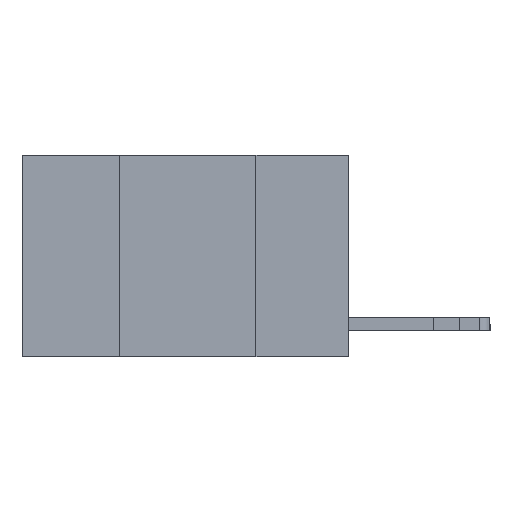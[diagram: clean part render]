
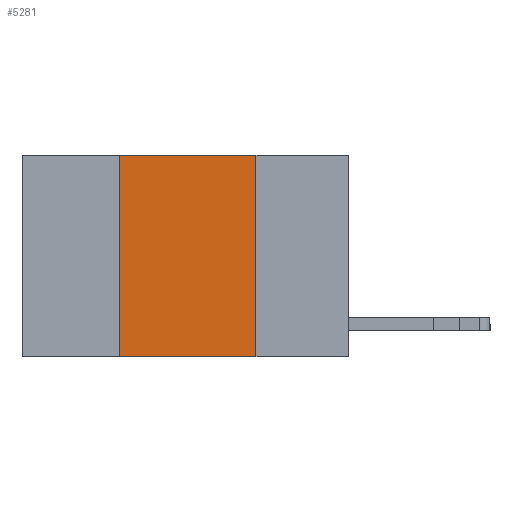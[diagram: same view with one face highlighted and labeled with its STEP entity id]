
A CAD part, left-side view. The second image highlights one B-rep face of the part: STEP entity #5281.
In plain terms, the highlighted planar face has unit normal (-1, 0, 0).
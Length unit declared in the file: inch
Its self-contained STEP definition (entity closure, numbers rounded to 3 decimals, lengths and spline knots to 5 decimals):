
#554 = CARTESIAN_POINT ( 'NONE',  ( 0., 0.42, 0. ) ) ;
#626 = CARTESIAN_POINT ( 'NONE',  ( 0., 0.42, 0. ) ) ;
#970 = ORIENTED_EDGE ( 'NONE', *, *, #9304, .F. ) ;
#1536 = DIRECTION ( 'NONE',  ( 0., -1., 0. ) ) ;
#3220 = EDGE_CURVE ( 'NONE', #19806, #18971, #14054, .T. ) ;
#4281 = LINE ( 'NONE', #626, #7802 ) ;
#4770 = ORIENTED_EDGE ( 'NONE', *, *, #15512, .T. ) ;
#5281 = ADVANCED_FACE ( 'NONE', ( #21952 ), #5828, .F. ) ;
#5628 = CARTESIAN_POINT ( 'NONE',  ( 0., 0.6, 0. ) ) ;
#5828 = PLANE ( 'NONE',  #13904 ) ;
#6828 = CARTESIAN_POINT ( 'NONE',  ( 0., 0.17, -0.37 ) ) ;
#6884 = VERTEX_POINT ( 'NONE', #6828 ) ;
#6937 = VECTOR ( 'NONE', #21202, 39.37008 ) ;
#7802 = VECTOR ( 'NONE', #11305, 39.37008 ) ;
#9304 = EDGE_CURVE ( 'NONE', #18971, #6884, #22130, .T. ) ;
#10269 = LINE ( 'NONE', #20995, #11437 ) ;
#10493 = EDGE_CURVE ( 'NONE', #11701, #19806, #4281, .T. ) ;
#10815 = ORIENTED_EDGE ( 'NONE', *, *, #3220, .F. ) ;
#11289 = CARTESIAN_POINT ( 'NONE',  ( 0., 0.17, 0. ) ) ;
#11305 = DIRECTION ( 'NONE',  ( 0., 0., 1. ) ) ;
#11437 = VECTOR ( 'NONE', #1536, 39.37008 ) ;
#11701 = VERTEX_POINT ( 'NONE', #17473 ) ;
#13904 = AXIS2_PLACEMENT_3D ( 'NONE', #20468, #15609, #16902 ) ;
#14054 = LINE ( 'NONE', #5628, #6937 ) ;
#15512 = EDGE_CURVE ( 'NONE', #11701, #6884, #10269, .T. ) ;
#15609 = DIRECTION ( 'NONE',  ( 1., 0., 0. ) ) ;
#15657 = ORIENTED_EDGE ( 'NONE', *, *, #10493, .F. ) ;
#16902 = DIRECTION ( 'NONE',  ( 0., 0., -1. ) ) ;
#17473 = CARTESIAN_POINT ( 'NONE',  ( 0., 0.42, -0.37 ) ) ;
#17775 = VECTOR ( 'NONE', #20189, 39.37008 ) ;
#18971 = VERTEX_POINT ( 'NONE', #11289 ) ;
#19707 = EDGE_LOOP ( 'NONE', ( #970, #10815, #15657, #4770 ) ) ;
#19806 = VERTEX_POINT ( 'NONE', #554 ) ;
#20189 = DIRECTION ( 'NONE',  ( 0., 0., -1. ) ) ;
#20468 = CARTESIAN_POINT ( 'NONE',  ( 0., 0.6, 0. ) ) ;
#20995 = CARTESIAN_POINT ( 'NONE',  ( 0., 0.6, -0.37 ) ) ;
#21202 = DIRECTION ( 'NONE',  ( 0., -1., 0. ) ) ;
#21952 = FACE_OUTER_BOUND ( 'NONE', #19707, .T. ) ;
#22130 = LINE ( 'NONE', #22252, #17775 ) ;
#22252 = CARTESIAN_POINT ( 'NONE',  ( 0., 0.17, 0. ) ) ;
